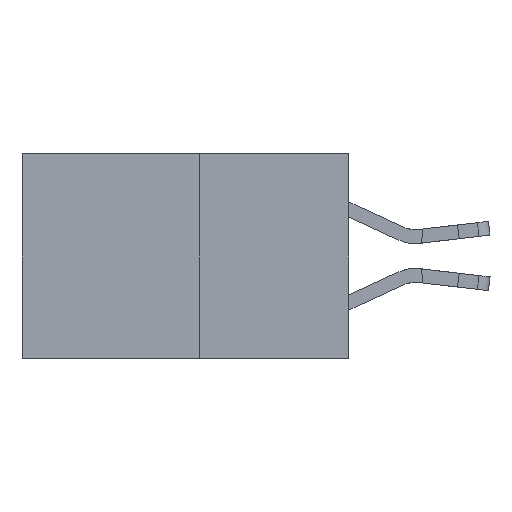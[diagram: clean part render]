
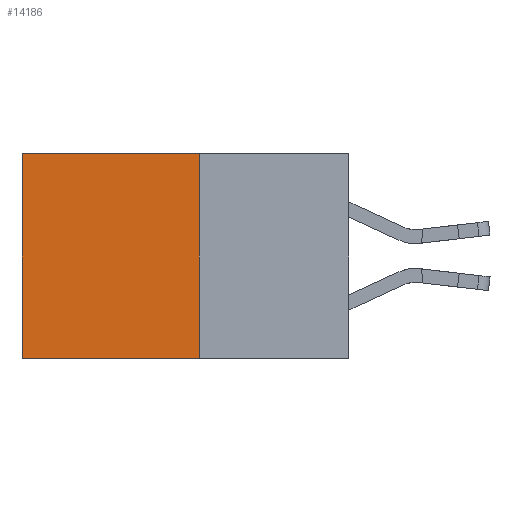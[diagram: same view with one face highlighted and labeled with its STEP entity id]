
A CAD part, left-side view. The second image highlights one B-rep face of the part: STEP entity #14186.
In plain terms, the highlighted planar face has unit normal (-1, 0, 0).
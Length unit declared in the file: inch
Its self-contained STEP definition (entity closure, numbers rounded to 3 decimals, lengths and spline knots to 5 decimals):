
#347 = DIRECTION ( 'NONE',  ( 0., 1., 0. ) ) ;
#1174 = CARTESIAN_POINT ( 'NONE',  ( 0.277, 0.27, -0.37 ) ) ;
#1323 = FACE_OUTER_BOUND ( 'NONE', #8947, .T. ) ;
#2066 = EDGE_CURVE ( 'NONE', #16626, #3573, #2942, .T. ) ;
#2236 = DIRECTION ( 'NONE',  ( 0., 0., -1. ) ) ;
#2288 = DIRECTION ( 'NONE',  ( 0., 1., 0. ) ) ;
#2355 = PLANE ( 'NONE',  #7926 ) ;
#2942 = LINE ( 'NONE', #1174, #13975 ) ;
#3142 = CARTESIAN_POINT ( 'NONE',  ( 0.277, 0.27, -0.37 ) ) ;
#3573 = VERTEX_POINT ( 'NONE', #3142 ) ;
#3969 = CARTESIAN_POINT ( 'NONE',  ( 0.277, 0.59, -0.37 ) ) ;
#4090 = ORIENTED_EDGE ( 'NONE', *, *, #2066, .F. ) ;
#5260 = DIRECTION ( 'NONE',  ( 0., 0., -1. ) ) ;
#5785 = CARTESIAN_POINT ( 'NONE',  ( 0.277, 0.27, 0. ) ) ;
#6715 = CARTESIAN_POINT ( 'NONE',  ( 0.277, 0.59, -0.37 ) ) ;
#6720 = LINE ( 'NONE', #11897, #13943 ) ;
#7926 = AXIS2_PLACEMENT_3D ( 'NONE', #12431, #13880, #5260 ) ;
#7930 = CARTESIAN_POINT ( 'NONE',  ( 0.277, 0.59, 0. ) ) ;
#8947 = EDGE_LOOP ( 'NONE', ( #14857, #17129, #4090, #18276 ) ) ;
#9429 = VECTOR ( 'NONE', #15384, 39.37008 ) ;
#9483 = LINE ( 'NONE', #12367, #16728 ) ;
#11588 = VERTEX_POINT ( 'NONE', #3969 ) ;
#11897 = CARTESIAN_POINT ( 'NONE',  ( 0.277, 0.27, 0. ) ) ;
#12130 = EDGE_CURVE ( 'NONE', #3573, #11588, #9483, .T. ) ;
#12367 = CARTESIAN_POINT ( 'NONE',  ( 0.277, 0.27, -0.37 ) ) ;
#12431 = CARTESIAN_POINT ( 'NONE',  ( 0.277, 0.27, -0.37 ) ) ;
#13284 = LINE ( 'NONE', #6715, #9429 ) ;
#13447 = EDGE_CURVE ( 'NONE', #18427, #11588, #13284, .T. ) ;
#13880 = DIRECTION ( 'NONE',  ( 1., 0., 0. ) ) ;
#13943 = VECTOR ( 'NONE', #347, 39.37008 ) ;
#13975 = VECTOR ( 'NONE', #2236, 39.37008 ) ;
#14186 = ADVANCED_FACE ( 'NONE', ( #1323 ), #2355, .F. ) ;
#14857 = ORIENTED_EDGE ( 'NONE', *, *, #13447, .T. ) ;
#15384 = DIRECTION ( 'NONE',  ( 0., 0., -1. ) ) ;
#16626 = VERTEX_POINT ( 'NONE', #5785 ) ;
#16728 = VECTOR ( 'NONE', #2288, 39.37008 ) ;
#17129 = ORIENTED_EDGE ( 'NONE', *, *, #12130, .F. ) ;
#17546 = EDGE_CURVE ( 'NONE', #16626, #18427, #6720, .T. ) ;
#18276 = ORIENTED_EDGE ( 'NONE', *, *, #17546, .T. ) ;
#18427 = VERTEX_POINT ( 'NONE', #7930 ) ;
